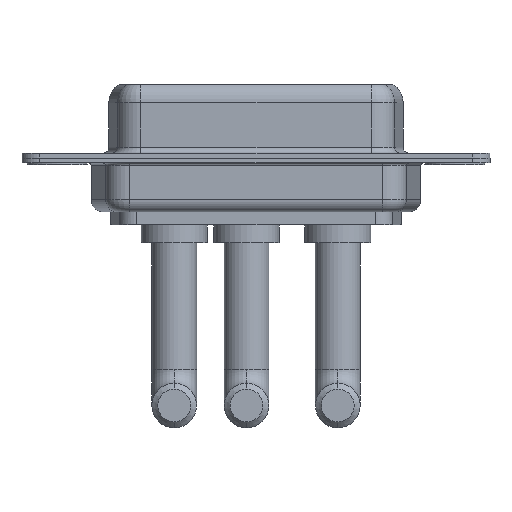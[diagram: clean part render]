
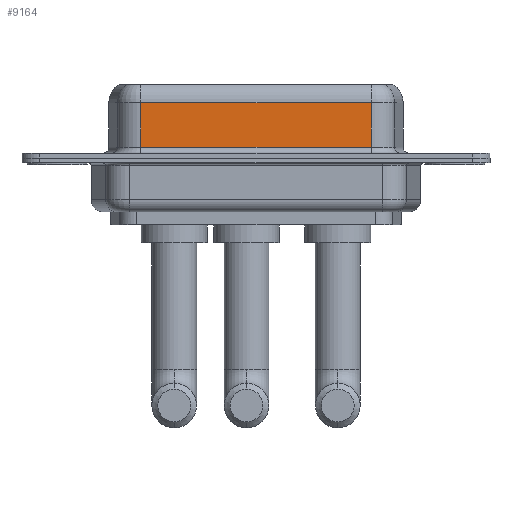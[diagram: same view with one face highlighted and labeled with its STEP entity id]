
A CAD part, front view. The second image highlights one B-rep face of the part: STEP entity #9164.
In plain terms, the highlighted planar face has unit normal (0, -1, 0).
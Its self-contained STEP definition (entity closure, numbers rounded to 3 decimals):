
#379 = VECTOR ( 'NONE', #2761, 1000. ) ;
#695 = ORIENTED_EDGE ( 'NONE', *, *, #10500, .T. ) ;
#939 = AXIS2_PLACEMENT_3D ( 'NONE', #3463, #11852, #6535 ) ;
#1185 = VERTEX_POINT ( 'NONE', #2429 ) ;
#1544 = VECTOR ( 'NONE', #1715, 1000. ) ;
#1715 = DIRECTION ( 'NONE',  ( 0., 0., -1. ) ) ;
#1740 = VECTOR ( 'NONE', #8243, 1000. ) ;
#1888 = ORIENTED_EDGE ( 'NONE', *, *, #11662, .T. ) ;
#2053 = DIRECTION ( 'NONE',  ( 1., 0., 0. ) ) ;
#2085 = CARTESIAN_POINT ( 'NONE',  ( 26.287, -3.95, 4.65 ) ) ;
#2429 = CARTESIAN_POINT ( 'NONE',  ( 7.013, -3.95, 0.9 ) ) ;
#2639 = LINE ( 'NONE', #10034, #1544 ) ;
#2761 = DIRECTION ( 'NONE',  ( -1., 0., 0. ) ) ;
#3080 = LINE ( 'NONE', #6827, #7576 ) ;
#3463 = CARTESIAN_POINT ( 'NONE',  ( 26.287, -3.95, 6.4 ) ) ;
#3527 = PLANE ( 'NONE',  #939 ) ;
#4072 = ORIENTED_EDGE ( 'NONE', *, *, #11813, .F. ) ;
#4282 = LINE ( 'NONE', #10884, #1740 ) ;
#5222 = VERTEX_POINT ( 'NONE', #7733 ) ;
#5637 = LINE ( 'NONE', #9324, #379 ) ;
#6289 = ORIENTED_EDGE ( 'NONE', *, *, #11924, .T. ) ;
#6535 = DIRECTION ( 'NONE',  ( 0., 0., 1. ) ) ;
#6827 = CARTESIAN_POINT ( 'NONE',  ( 26.287, -3.95, 0.9 ) ) ;
#7576 = VECTOR ( 'NONE', #2053, 1000. ) ;
#7733 = CARTESIAN_POINT ( 'NONE',  ( 7.013, -3.95, 4.65 ) ) ;
#8243 = DIRECTION ( 'NONE',  ( 0., 0., -1. ) ) ;
#9164 = ADVANCED_FACE ( 'NONE', ( #9956 ), #3527, .F. ) ;
#9324 = CARTESIAN_POINT ( 'NONE',  ( 26.287, -3.95, 4.65 ) ) ;
#9728 = CARTESIAN_POINT ( 'NONE',  ( 26.287, -3.95, 0.9 ) ) ;
#9909 = EDGE_LOOP ( 'NONE', ( #4072, #6289, #1888, #695 ) ) ;
#9956 = FACE_OUTER_BOUND ( 'NONE', #9909, .T. ) ;
#10034 = CARTESIAN_POINT ( 'NONE',  ( 26.287, -3.95, 6.4 ) ) ;
#10500 = EDGE_CURVE ( 'NONE', #1185, #11545, #3080, .T. ) ;
#10884 = CARTESIAN_POINT ( 'NONE',  ( 7.013, -3.95, 6.4 ) ) ;
#11429 = VERTEX_POINT ( 'NONE', #2085 ) ;
#11545 = VERTEX_POINT ( 'NONE', #9728 ) ;
#11662 = EDGE_CURVE ( 'NONE', #5222, #1185, #4282, .T. ) ;
#11813 = EDGE_CURVE ( 'NONE', #11429, #11545, #2639, .T. ) ;
#11852 = DIRECTION ( 'NONE',  ( 0., 1., 0. ) ) ;
#11924 = EDGE_CURVE ( 'NONE', #11429, #5222, #5637, .T. ) ;
